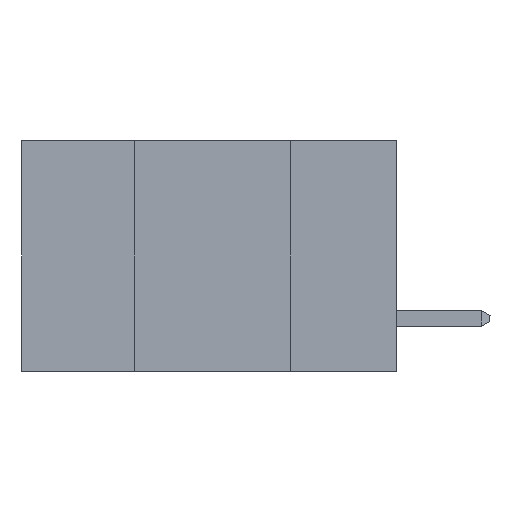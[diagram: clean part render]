
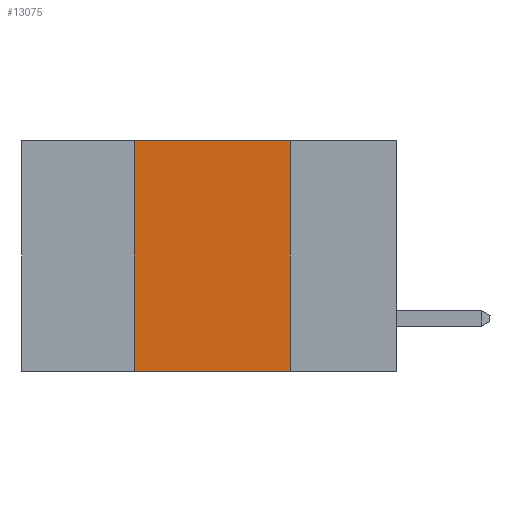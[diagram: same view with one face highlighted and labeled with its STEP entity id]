
A CAD part, left-side view. The second image highlights one B-rep face of the part: STEP entity #13075.
In plain terms, the highlighted planar face has unit normal (-1, 0, 0).
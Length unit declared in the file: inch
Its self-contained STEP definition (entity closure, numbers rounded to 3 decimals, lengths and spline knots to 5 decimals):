
#81 = VECTOR ( 'NONE', #1264, 39.37008 ) ;
#316 = ORIENTED_EDGE ( 'NONE', *, *, #7892, .F. ) ;
#327 = VERTEX_POINT ( 'NONE', #5389 ) ;
#624 = EDGE_CURVE ( 'NONE', #1157, #15097, #5309, .T. ) ;
#800 = DIRECTION ( 'NONE',  ( 0., -1., 0. ) ) ;
#1157 = VERTEX_POINT ( 'NONE', #2652 ) ;
#1264 = DIRECTION ( 'NONE',  ( 0., -1., 0. ) ) ;
#2026 = EDGE_CURVE ( 'NONE', #16169, #327, #5883, .T. ) ;
#2259 = ORIENTED_EDGE ( 'NONE', *, *, #2026, .T. ) ;
#2652 = CARTESIAN_POINT ( 'NONE',  ( 0., 0.42, 0. ) ) ;
#3375 = DIRECTION ( 'NONE',  ( 0., 0., -1. ) ) ;
#3706 = CARTESIAN_POINT ( 'NONE',  ( 0., 0.42, 0. ) ) ;
#3771 = ORIENTED_EDGE ( 'NONE', *, *, #16516, .F. ) ;
#3872 = VECTOR ( 'NONE', #3375, 39.37008 ) ;
#4081 = LINE ( 'NONE', #12567, #3872 ) ;
#4150 = AXIS2_PLACEMENT_3D ( 'NONE', #7338, #8629, #9904 ) ;
#5309 = LINE ( 'NONE', #15136, #81 ) ;
#5389 = CARTESIAN_POINT ( 'NONE',  ( 0., 0.17, -0.37 ) ) ;
#5883 = LINE ( 'NONE', #8909, #13482 ) ;
#6045 = PLANE ( 'NONE',  #4150 ) ;
#6225 = DIRECTION ( 'NONE',  ( 0., 0., 1. ) ) ;
#6327 = ORIENTED_EDGE ( 'NONE', *, *, #624, .F. ) ;
#7338 = CARTESIAN_POINT ( 'NONE',  ( 0., 0.6, 0. ) ) ;
#7892 = EDGE_CURVE ( 'NONE', #16169, #1157, #16090, .T. ) ;
#8022 = FACE_OUTER_BOUND ( 'NONE', #12340, .T. ) ;
#8629 = DIRECTION ( 'NONE',  ( 1., 0., 0. ) ) ;
#8909 = CARTESIAN_POINT ( 'NONE',  ( 0., 0.6, -0.37 ) ) ;
#9187 = CARTESIAN_POINT ( 'NONE',  ( 0., 0.17, 0. ) ) ;
#9904 = DIRECTION ( 'NONE',  ( 0., 0., -1. ) ) ;
#12340 = EDGE_LOOP ( 'NONE', ( #3771, #6327, #316, #2259 ) ) ;
#12567 = CARTESIAN_POINT ( 'NONE',  ( 0., 0.17, 0. ) ) ;
#12669 = VECTOR ( 'NONE', #6225, 39.37008 ) ;
#13075 = ADVANCED_FACE ( 'NONE', ( #8022 ), #6045, .F. ) ;
#13482 = VECTOR ( 'NONE', #800, 39.37008 ) ;
#13889 = CARTESIAN_POINT ( 'NONE',  ( 0., 0.42, -0.37 ) ) ;
#15097 = VERTEX_POINT ( 'NONE', #9187 ) ;
#15136 = CARTESIAN_POINT ( 'NONE',  ( 0., 0.6, 0. ) ) ;
#16090 = LINE ( 'NONE', #3706, #12669 ) ;
#16169 = VERTEX_POINT ( 'NONE', #13889 ) ;
#16516 = EDGE_CURVE ( 'NONE', #15097, #327, #4081, .T. ) ;
